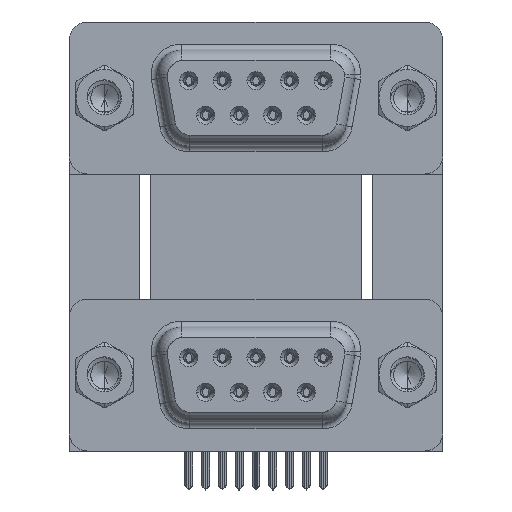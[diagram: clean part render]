
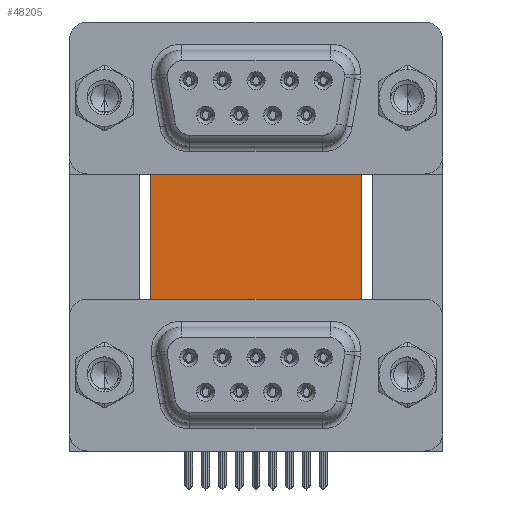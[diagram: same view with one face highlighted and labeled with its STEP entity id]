
A CAD part, top view. The second image highlights one B-rep face of the part: STEP entity #48205.
In plain terms, the highlighted planar face has unit normal (0, 0, 1).
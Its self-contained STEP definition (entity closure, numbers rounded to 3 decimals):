
#718 = EDGE_CURVE ( 'NONE', #42150, #45856, #9430, .T. ) ;
#1321 = VERTEX_POINT ( 'NONE', #9253 ) ;
#2229 = DIRECTION ( 'NONE',  ( 0., 1., 0. ) ) ;
#2747 = LINE ( 'NONE', #32416, #7711 ) ;
#3334 = CARTESIAN_POINT ( 'NONE',  ( 22.59, -4.635, -12. ) ) ;
#4512 = LINE ( 'NONE', #42190, #46823 ) ;
#5103 = VERTEX_POINT ( 'NONE', #29123 ) ;
#5992 = LINE ( 'NONE', #9976, #42539 ) ;
#6169 = DIRECTION ( 'NONE',  ( 1., 0., 0. ) ) ;
#6336 = CARTESIAN_POINT ( 'NONE',  ( 3.79, 16.585, -12. ) ) ;
#7075 = EDGE_CURVE ( 'NONE', #5103, #42150, #35040, .T. ) ;
#7277 = ORIENTED_EDGE ( 'NONE', *, *, #38636, .T. ) ;
#7711 = VECTOR ( 'NONE', #21681, 1000. ) ;
#7734 = EDGE_CURVE ( 'NONE', #16551, #17069, #2747, .T. ) ;
#8486 = VECTOR ( 'NONE', #29259, 1000. ) ;
#9253 = CARTESIAN_POINT ( 'NONE',  ( 2.9, -4.635, -12. ) ) ;
#9430 = LINE ( 'NONE', #16891, #19057 ) ;
#9619 = CARTESIAN_POINT ( 'NONE',  ( 2.4, -4.635, -12. ) ) ;
#9976 = CARTESIAN_POINT ( 'NONE',  ( 2.9, -3.735, -12. ) ) ;
#10121 = EDGE_CURVE ( 'NONE', #46661, #1321, #21349, .T. ) ;
#13103 = LINE ( 'NONE', #9619, #24252 ) ;
#13340 = DIRECTION ( 'NONE',  ( -0.336, -0.942, 0. ) ) ;
#13414 = DIRECTION ( 'NONE',  ( 1., 0., 0. ) ) ;
#14628 = CARTESIAN_POINT ( 'NONE',  ( 2.9, -4.635, -12. ) ) ;
#15127 = DIRECTION ( 'NONE',  ( 0., 0., -1. ) ) ;
#16397 = ORIENTED_EDGE ( 'NONE', *, *, #43378, .T. ) ;
#16551 = VERTEX_POINT ( 'NONE', #33379 ) ;
#16891 = CARTESIAN_POINT ( 'NONE',  ( 21.2, 16.585, -12. ) ) ;
#16906 = CARTESIAN_POINT ( 'NONE',  ( 22.09, -4.635, -12. ) ) ;
#17069 = VERTEX_POINT ( 'NONE', #38308 ) ;
#17422 = VERTEX_POINT ( 'NONE', #46467 ) ;
#18116 = ORIENTED_EDGE ( 'NONE', *, *, #45056, .T. ) ;
#18483 = ORIENTED_EDGE ( 'NONE', *, *, #18832, .T. ) ;
#18637 = VECTOR ( 'NONE', #19580, 1000. ) ;
#18832 = EDGE_CURVE ( 'NONE', #29447, #35417, #28387, .T. ) ;
#18851 = VECTOR ( 'NONE', #48485, 1000. ) ;
#19057 = VECTOR ( 'NONE', #44106, 1000. ) ;
#19580 = DIRECTION ( 'NONE',  ( 1., 0., 0. ) ) ;
#19590 = FACE_OUTER_BOUND ( 'NONE', #29735, .T. ) ;
#20772 = ORIENTED_EDGE ( 'NONE', *, *, #7075, .F. ) ;
#20841 = EDGE_CURVE ( 'NONE', #5103, #17422, #44995, .T. ) ;
#21349 = LINE ( 'NONE', #14628, #45567 ) ;
#21681 = DIRECTION ( 'NONE',  ( 1., 0., 0. ) ) ;
#22026 = LINE ( 'NONE', #3334, #8486 ) ;
#22598 = PLANE ( 'NONE',  #32524 ) ;
#24252 = VECTOR ( 'NONE', #13340, 1000. ) ;
#25784 = CARTESIAN_POINT ( 'NONE',  ( 21.2, -0.735, -12. ) ) ;
#26187 = CARTESIAN_POINT ( 'NONE',  ( 21.2, 16.585, -12. ) ) ;
#26575 = CARTESIAN_POINT ( 'NONE',  ( 3.79, 16.585, -12. ) ) ;
#27066 = CARTESIAN_POINT ( 'NONE',  ( 3.79, 16.585, -12. ) ) ;
#27504 = VECTOR ( 'NONE', #13414, 1000. ) ;
#28387 = LINE ( 'NONE', #16906, #27504 ) ;
#29123 = CARTESIAN_POINT ( 'NONE',  ( 3.79, 16.585, -12. ) ) ;
#29259 = DIRECTION ( 'NONE',  ( -0.336, 0.942, 0. ) ) ;
#29447 = VERTEX_POINT ( 'NONE', #39184 ) ;
#29735 = EDGE_LOOP ( 'NONE', ( #35353, #18116, #18483, #16397, #36018, #20772, #35961, #45387, #31876, #7277 ) ) ;
#30411 = CARTESIAN_POINT ( 'NONE',  ( 2.4, -4.635, -12. ) ) ;
#31876 = ORIENTED_EDGE ( 'NONE', *, *, #10121, .T. ) ;
#32416 = CARTESIAN_POINT ( 'NONE',  ( 3.79, -3.735, -12. ) ) ;
#32524 = AXIS2_PLACEMENT_3D ( 'NONE', #27066, #15127, #34323 ) ;
#33379 = CARTESIAN_POINT ( 'NONE',  ( 2.9, -3.735, -12. ) ) ;
#34323 = DIRECTION ( 'NONE',  ( -1., 0., 0. ) ) ;
#34674 = DIRECTION ( 'NONE',  ( 0., -1., 0. ) ) ;
#35040 = LINE ( 'NONE', #26575, #18637 ) ;
#35353 = ORIENTED_EDGE ( 'NONE', *, *, #7734, .T. ) ;
#35417 = VERTEX_POINT ( 'NONE', #46404 ) ;
#35961 = ORIENTED_EDGE ( 'NONE', *, *, #20841, .T. ) ;
#36018 = ORIENTED_EDGE ( 'NONE', *, *, #718, .F. ) ;
#38308 = CARTESIAN_POINT ( 'NONE',  ( 22.09, -3.735, -12. ) ) ;
#38636 = EDGE_CURVE ( 'NONE', #1321, #16551, #5992, .T. ) ;
#39184 = CARTESIAN_POINT ( 'NONE',  ( 22.09, -4.635, -12. ) ) ;
#40041 = EDGE_CURVE ( 'NONE', #17422, #46661, #13103, .T. ) ;
#42150 = VERTEX_POINT ( 'NONE', #26187 ) ;
#42190 = CARTESIAN_POINT ( 'NONE',  ( 22.09, -3.735, -12. ) ) ;
#42539 = VECTOR ( 'NONE', #2229, 1000. ) ;
#43378 = EDGE_CURVE ( 'NONE', #35417, #45856, #22026, .T. ) ;
#44106 = DIRECTION ( 'NONE',  ( 0., -1., 0. ) ) ;
#44995 = LINE ( 'NONE', #6336, #18851 ) ;
#45056 = EDGE_CURVE ( 'NONE', #17069, #29447, #4512, .T. ) ;
#45387 = ORIENTED_EDGE ( 'NONE', *, *, #40041, .T. ) ;
#45567 = VECTOR ( 'NONE', #6169, 1000. ) ;
#45856 = VERTEX_POINT ( 'NONE', #25784 ) ;
#46404 = CARTESIAN_POINT ( 'NONE',  ( 22.59, -4.635, -12. ) ) ;
#46467 = CARTESIAN_POINT ( 'NONE',  ( 3.79, -0.735, -12. ) ) ;
#46661 = VERTEX_POINT ( 'NONE', #30411 ) ;
#46823 = VECTOR ( 'NONE', #34674, 1000. ) ;
#48205 = ADVANCED_FACE ( 'NONE', ( #19590 ), #22598, .F. ) ;
#48485 = DIRECTION ( 'NONE',  ( 0., -1., 0. ) ) ;
